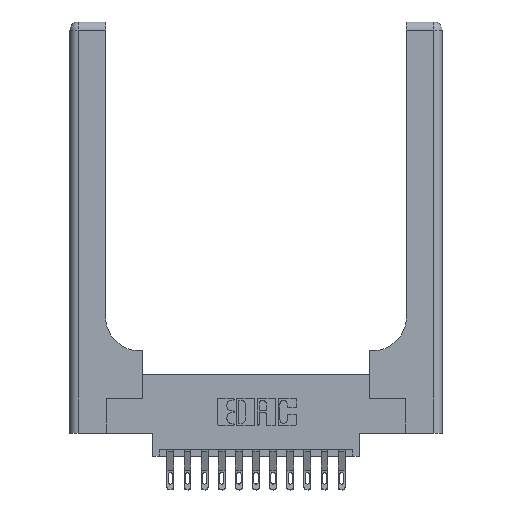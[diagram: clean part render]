
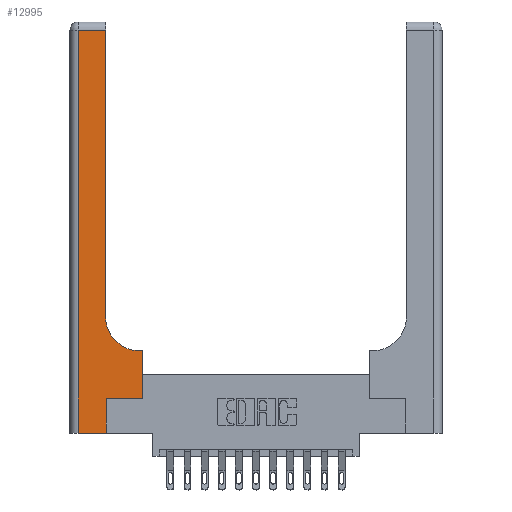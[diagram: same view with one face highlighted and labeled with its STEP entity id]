
A CAD part, top view. The second image highlights one B-rep face of the part: STEP entity #12995.
In plain terms, the highlighted planar face has unit normal (0, 0, 1).
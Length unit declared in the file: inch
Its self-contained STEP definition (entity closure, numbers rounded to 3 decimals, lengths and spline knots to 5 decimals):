
#211 = VECTOR ( 'NONE', #6683, 39.37008 ) ;
#240 = CARTESIAN_POINT ( 'NONE',  ( 0.528, 0.6, 0.37 ) ) ;
#434 = EDGE_CURVE ( 'NONE', #15507, #13607, #12601, .T. ) ;
#538 = EDGE_CURVE ( 'NONE', #7535, #10184, #5136, .T. ) ;
#548 = DIRECTION ( 'NONE',  ( 0., 1., 0. ) ) ;
#654 = CARTESIAN_POINT ( 'NONE',  ( 0.06, 0., 0.37 ) ) ;
#720 = ORIENTED_EDGE ( 'NONE', *, *, #10350, .T. ) ;
#1090 = LINE ( 'NONE', #6458, #4836 ) ;
#1295 = DIRECTION ( 'NONE',  ( 0., 1., 0. ) ) ;
#1688 = CARTESIAN_POINT ( 'NONE',  ( 0.265, 0.25, 0.37 ) ) ;
#1878 = CARTESIAN_POINT ( 'NONE',  ( 0.265, 0., 0.37 ) ) ;
#1910 = CARTESIAN_POINT ( 'NONE',  ( 0.51, 0.85, 0.37 ) ) ;
#2270 = EDGE_CURVE ( 'NONE', #13607, #9830, #5581, .T. ) ;
#2624 = LINE ( 'NONE', #14370, #8089 ) ;
#2805 = CARTESIAN_POINT ( 'NONE',  ( 0.528, 0.25, 0.37 ) ) ;
#2830 = AXIS2_PLACEMENT_3D ( 'NONE', #13887, #5017, #10408 ) ;
#3095 = VERTEX_POINT ( 'NONE', #240 ) ;
#3848 = LINE ( 'NONE', #5250, #9776 ) ;
#4315 = DIRECTION ( 'NONE',  ( -1., 0., 0. ) ) ;
#4471 = DIRECTION ( 'NONE',  ( 0., 1., 0. ) ) ;
#4538 = CARTESIAN_POINT ( 'NONE',  ( 0.51, 0.6, 0.37 ) ) ;
#4653 = DIRECTION ( 'NONE',  ( 1., 0., 0. ) ) ;
#4836 = VECTOR ( 'NONE', #16276, 39.37008 ) ;
#5017 = DIRECTION ( 'NONE',  ( 0., 0., -1. ) ) ;
#5136 = CIRCLE ( 'NONE', #9116, 0.25 ) ;
#5148 = ORIENTED_EDGE ( 'NONE', *, *, #16280, .T. ) ;
#5250 = CARTESIAN_POINT ( 'NONE',  ( 0.265, 0.25, 0.37 ) ) ;
#5581 = LINE ( 'NONE', #10996, #8371 ) ;
#6263 = ORIENTED_EDGE ( 'NONE', *, *, #8931, .T. ) ;
#6363 = ORIENTED_EDGE ( 'NONE', *, *, #10152, .T. ) ;
#6458 = CARTESIAN_POINT ( 'NONE',  ( 0.26, 0.6, 0.37 ) ) ;
#6683 = DIRECTION ( 'NONE',  ( 1., 0., 0. ) ) ;
#7057 = PLANE ( 'NONE',  #2830 ) ;
#7080 = VERTEX_POINT ( 'NONE', #13829 ) ;
#7535 = VERTEX_POINT ( 'NONE', #4538 ) ;
#7622 = ORIENTED_EDGE ( 'NONE', *, *, #8691, .T. ) ;
#8040 = CARTESIAN_POINT ( 'NONE',  ( 0.26, 0.85, 0.37 ) ) ;
#8089 = VECTOR ( 'NONE', #1295, 39.37008 ) ;
#8278 = ORIENTED_EDGE ( 'NONE', *, *, #17146, .T. ) ;
#8371 = VECTOR ( 'NONE', #15113, 39.37008 ) ;
#8691 = EDGE_CURVE ( 'NONE', #11724, #3095, #14891, .T. ) ;
#8931 = EDGE_CURVE ( 'NONE', #15042, #11724, #3848, .T. ) ;
#9116 = AXIS2_PLACEMENT_3D ( 'NONE', #1910, #10400, #4653 ) ;
#9756 = LINE ( 'NONE', #1878, #10931 ) ;
#9776 = VECTOR ( 'NONE', #17077, 39.37008 ) ;
#9830 = VERTEX_POINT ( 'NONE', #654 ) ;
#10117 = CARTESIAN_POINT ( 'NONE',  ( 0.26, 2.94, 0.37 ) ) ;
#10152 = EDGE_CURVE ( 'NONE', #7080, #15042, #9756, .T. ) ;
#10184 = VERTEX_POINT ( 'NONE', #8040 ) ;
#10350 = EDGE_CURVE ( 'NONE', #10184, #15507, #2624, .T. ) ;
#10400 = DIRECTION ( 'NONE',  ( 0., 0., -1. ) ) ;
#10408 = DIRECTION ( 'NONE',  ( -1., 0., 0. ) ) ;
#10615 = VECTOR ( 'NONE', #4471, 39.37008 ) ;
#10931 = VECTOR ( 'NONE', #548, 39.37008 ) ;
#10996 = CARTESIAN_POINT ( 'NONE',  ( 0.06, 3., 0.37 ) ) ;
#11724 = VERTEX_POINT ( 'NONE', #14429 ) ;
#11744 = FACE_OUTER_BOUND ( 'NONE', #13150, .T. ) ;
#11826 = LINE ( 'NONE', #17358, #211 ) ;
#12176 = VECTOR ( 'NONE', #4315, 39.37008 ) ;
#12601 = LINE ( 'NONE', #16403, #12176 ) ;
#12995 = ADVANCED_FACE ( 'NONE', ( #11744 ), #7057, .F. ) ;
#13150 = EDGE_LOOP ( 'NONE', ( #720, #16144, #17040, #8278, #6363, #6263, #7622, #5148, #15606 ) ) ;
#13607 = VERTEX_POINT ( 'NONE', #15520 ) ;
#13829 = CARTESIAN_POINT ( 'NONE',  ( 0.265, 0., 0.37 ) ) ;
#13887 = CARTESIAN_POINT ( 'NONE',  ( 0., 3., 0.37 ) ) ;
#14370 = CARTESIAN_POINT ( 'NONE',  ( 0.26, 3., 0.37 ) ) ;
#14429 = CARTESIAN_POINT ( 'NONE',  ( 0.528, 0.25, 0.37 ) ) ;
#14891 = LINE ( 'NONE', #2805, #10615 ) ;
#15042 = VERTEX_POINT ( 'NONE', #1688 ) ;
#15113 = DIRECTION ( 'NONE',  ( 0., -1., 0. ) ) ;
#15507 = VERTEX_POINT ( 'NONE', #10117 ) ;
#15520 = CARTESIAN_POINT ( 'NONE',  ( 0.06, 2.94, 0.37 ) ) ;
#15606 = ORIENTED_EDGE ( 'NONE', *, *, #538, .T. ) ;
#16144 = ORIENTED_EDGE ( 'NONE', *, *, #434, .T. ) ;
#16276 = DIRECTION ( 'NONE',  ( -1., 0., 0. ) ) ;
#16280 = EDGE_CURVE ( 'NONE', #3095, #7535, #1090, .T. ) ;
#16403 = CARTESIAN_POINT ( 'NONE',  ( 0., 2.94, 0.37 ) ) ;
#17040 = ORIENTED_EDGE ( 'NONE', *, *, #2270, .T. ) ;
#17077 = DIRECTION ( 'NONE',  ( 1., 0., 0. ) ) ;
#17146 = EDGE_CURVE ( 'NONE', #9830, #7080, #11826, .T. ) ;
#17358 = CARTESIAN_POINT ( 'NONE',  ( 0., 0., 0.37 ) ) ;
